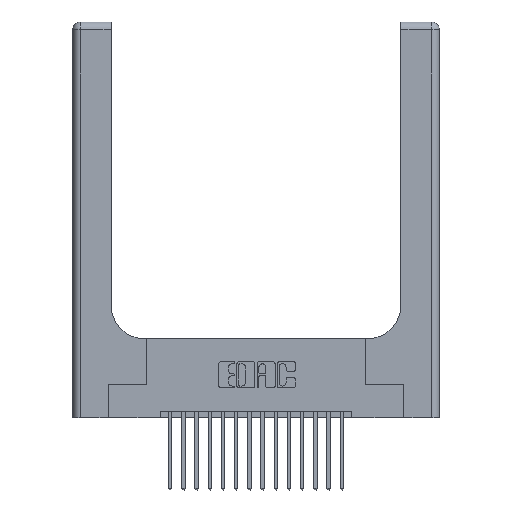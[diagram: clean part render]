
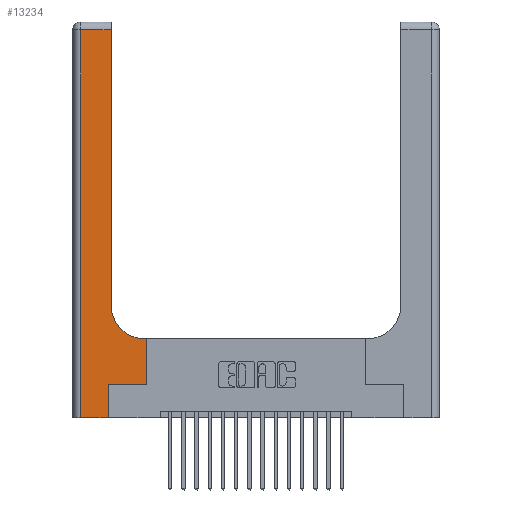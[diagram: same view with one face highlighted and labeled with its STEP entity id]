
A CAD part, top view. The second image highlights one B-rep face of the part: STEP entity #13234.
In plain terms, the highlighted planar face has unit normal (0, 0, 1).
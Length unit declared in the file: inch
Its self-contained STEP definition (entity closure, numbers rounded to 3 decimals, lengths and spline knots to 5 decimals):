
#37 = EDGE_CURVE ( 'NONE', #12332, #6432, #5704, .T. ) ;
#204 = LINE ( 'NONE', #7505, #8167 ) ;
#284 = CARTESIAN_POINT ( 'NONE',  ( 0.5585, 0.25, 0.37 ) ) ;
#319 = EDGE_CURVE ( 'NONE', #8413, #12332, #12713, .T. ) ;
#492 = DIRECTION ( 'NONE',  ( -1., 0., 0. ) ) ;
#531 = VERTEX_POINT ( 'NONE', #3267 ) ;
#1022 = CARTESIAN_POINT ( 'NONE',  ( 0.269, 0., 0.37 ) ) ;
#1089 = AXIS2_PLACEMENT_3D ( 'NONE', #3632, #9999, #492 ) ;
#1097 = CARTESIAN_POINT ( 'NONE',  ( 0.06, 0., 0.37 ) ) ;
#1198 = DIRECTION ( 'NONE',  ( 0., 1., 0. ) ) ;
#1741 = FACE_OUTER_BOUND ( 'NONE', #2450, .T. ) ;
#2409 = LINE ( 'NONE', #18212, #15284 ) ;
#2450 = EDGE_LOOP ( 'NONE', ( #15381, #6093, #13156, #8543, #2724, #4441, #9015, #14419, #8936 ) ) ;
#2724 = ORIENTED_EDGE ( 'NONE', *, *, #18483, .T. ) ;
#2750 = LINE ( 'NONE', #8426, #6494 ) ;
#2849 = VERTEX_POINT ( 'NONE', #5524 ) ;
#3267 = CARTESIAN_POINT ( 'NONE',  ( 0.2915, 0.85, 0.37 ) ) ;
#3597 = CARTESIAN_POINT ( 'NONE',  ( 0.5415, 0.6, 0.37 ) ) ;
#3632 = CARTESIAN_POINT ( 'NONE',  ( 0., 3., 0.37 ) ) ;
#4441 = ORIENTED_EDGE ( 'NONE', *, *, #7233, .T. ) ;
#4498 = DIRECTION ( 'NONE',  ( 1., 0., 0. ) ) ;
#5057 = DIRECTION ( 'NONE',  ( 0., 0., -1. ) ) ;
#5201 = VECTOR ( 'NONE', #11725, 39.37008 ) ;
#5524 = CARTESIAN_POINT ( 'NONE',  ( 0.269, 0.25, 0.37 ) ) ;
#5704 = LINE ( 'NONE', #11635, #5201 ) ;
#6093 = ORIENTED_EDGE ( 'NONE', *, *, #12692, .T. ) ;
#6426 = VECTOR ( 'NONE', #17803, 39.37008 ) ;
#6432 = VERTEX_POINT ( 'NONE', #1022 ) ;
#6494 = VECTOR ( 'NONE', #17575, 39.37008 ) ;
#6631 = CARTESIAN_POINT ( 'NONE',  ( 0.06, 3., 0.37 ) ) ;
#6707 = DIRECTION ( 'NONE',  ( 0., -1., 0. ) ) ;
#7099 = CARTESIAN_POINT ( 'NONE',  ( 0.2915, 0.6, 0.37 ) ) ;
#7233 = EDGE_CURVE ( 'NONE', #2849, #15061, #15221, .T. ) ;
#7505 = CARTESIAN_POINT ( 'NONE',  ( 0.269, 0., 0.37 ) ) ;
#8167 = VECTOR ( 'NONE', #1198, 39.37008 ) ;
#8413 = VERTEX_POINT ( 'NONE', #11894 ) ;
#8426 = CARTESIAN_POINT ( 'NONE',  ( 0., 2.94, 0.37 ) ) ;
#8543 = ORIENTED_EDGE ( 'NONE', *, *, #37, .T. ) ;
#8728 = LINE ( 'NONE', #10374, #12348 ) ;
#8844 = VERTEX_POINT ( 'NONE', #15627 ) ;
#8936 = ORIENTED_EDGE ( 'NONE', *, *, #11306, .T. ) ;
#9015 = ORIENTED_EDGE ( 'NONE', *, *, #15902, .T. ) ;
#9181 = DIRECTION ( 'NONE',  ( 0., 1., 0. ) ) ;
#9621 = VECTOR ( 'NONE', #6707, 39.37008 ) ;
#9831 = AXIS2_PLACEMENT_3D ( 'NONE', #14292, #5057, #15801 ) ;
#9999 = DIRECTION ( 'NONE',  ( 0., 0., -1. ) ) ;
#10374 = CARTESIAN_POINT ( 'NONE',  ( 0.5585, 0.25, 0.37 ) ) ;
#10604 = VERTEX_POINT ( 'NONE', #3597 ) ;
#10612 = LINE ( 'NONE', #7099, #6426 ) ;
#11232 = VECTOR ( 'NONE', #4498, 39.37008 ) ;
#11306 = EDGE_CURVE ( 'NONE', #10604, #531, #19143, .T. ) ;
#11635 = CARTESIAN_POINT ( 'NONE',  ( 0., 0., 0.37 ) ) ;
#11725 = DIRECTION ( 'NONE',  ( 1., 0., 0. ) ) ;
#11894 = CARTESIAN_POINT ( 'NONE',  ( 0.06, 2.94, 0.37 ) ) ;
#12332 = VERTEX_POINT ( 'NONE', #1097 ) ;
#12348 = VECTOR ( 'NONE', #17922, 39.37008 ) ;
#12692 = EDGE_CURVE ( 'NONE', #18394, #8413, #2750, .T. ) ;
#12713 = LINE ( 'NONE', #6631, #9621 ) ;
#13156 = ORIENTED_EDGE ( 'NONE', *, *, #319, .T. ) ;
#13234 = ADVANCED_FACE ( 'NONE', ( #1741 ), #18963, .F. ) ;
#14292 = CARTESIAN_POINT ( 'NONE',  ( 0.5415, 0.85, 0.37 ) ) ;
#14419 = ORIENTED_EDGE ( 'NONE', *, *, #18831, .T. ) ;
#14765 = EDGE_CURVE ( 'NONE', #531, #18394, #2409, .T. ) ;
#15061 = VERTEX_POINT ( 'NONE', #284 ) ;
#15221 = LINE ( 'NONE', #16717, #11232 ) ;
#15284 = VECTOR ( 'NONE', #9181, 39.37008 ) ;
#15381 = ORIENTED_EDGE ( 'NONE', *, *, #14765, .T. ) ;
#15627 = CARTESIAN_POINT ( 'NONE',  ( 0.5585, 0.6, 0.37 ) ) ;
#15801 = DIRECTION ( 'NONE',  ( 1., 0., 0. ) ) ;
#15902 = EDGE_CURVE ( 'NONE', #15061, #8844, #8728, .T. ) ;
#16271 = CARTESIAN_POINT ( 'NONE',  ( 0.2915, 2.94, 0.37 ) ) ;
#16717 = CARTESIAN_POINT ( 'NONE',  ( 0.269, 0.25, 0.37 ) ) ;
#17575 = DIRECTION ( 'NONE',  ( -1., 0., 0. ) ) ;
#17803 = DIRECTION ( 'NONE',  ( -1., 0., 0. ) ) ;
#17922 = DIRECTION ( 'NONE',  ( 0., 1., 0. ) ) ;
#18212 = CARTESIAN_POINT ( 'NONE',  ( 0.2915, 3., 0.37 ) ) ;
#18394 = VERTEX_POINT ( 'NONE', #16271 ) ;
#18483 = EDGE_CURVE ( 'NONE', #6432, #2849, #204, .T. ) ;
#18831 = EDGE_CURVE ( 'NONE', #8844, #10604, #10612, .T. ) ;
#18963 = PLANE ( 'NONE',  #1089 ) ;
#19143 = CIRCLE ( 'NONE', #9831, 0.25 ) ;
